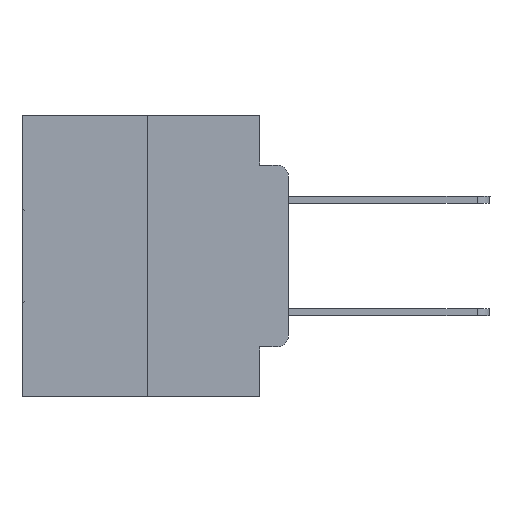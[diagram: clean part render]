
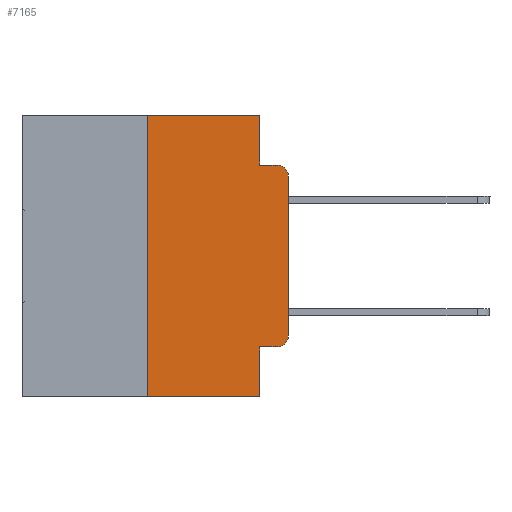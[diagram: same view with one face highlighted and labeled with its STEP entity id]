
A CAD part, left-side view. The second image highlights one B-rep face of the part: STEP entity #7165.
In plain terms, the highlighted planar face has unit normal (-1, 0, 0).
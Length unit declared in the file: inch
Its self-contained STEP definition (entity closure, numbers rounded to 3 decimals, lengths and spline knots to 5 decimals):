
#627 = CARTESIAN_POINT ( 'NONE',  ( 0., 0.25, 0. ) ) ;
#850 = DIRECTION ( 'NONE',  ( 0., 0., -1. ) ) ;
#1163 = LINE ( 'NONE', #29042, #15254 ) ;
#1243 = CARTESIAN_POINT ( 'NONE',  ( 0., 0., 0. ) ) ;
#1425 = DIRECTION ( 'NONE',  ( 1., 0., 0. ) ) ;
#1754 = VERTEX_POINT ( 'NONE', #24150 ) ;
#1997 = ORIENTED_EDGE ( 'NONE', *, *, #19515, .F. ) ;
#2080 = DIRECTION ( 'NONE',  ( 0., 0., 1. ) ) ;
#2230 = VERTEX_POINT ( 'NONE', #25196 ) ;
#2338 = ORIENTED_EDGE ( 'NONE', *, *, #7699, .T. ) ;
#2476 = LINE ( 'NONE', #18735, #23061 ) ;
#3043 = VERTEX_POINT ( 'NONE', #29175 ) ;
#3356 = VERTEX_POINT ( 'NONE', #10495 ) ;
#3398 = VECTOR ( 'NONE', #15623, 39.37008 ) ;
#3564 = LINE ( 'NONE', #5246, #29023 ) ;
#3790 = FACE_OUTER_BOUND ( 'NONE', #11510, .T. ) ;
#3826 = PLANE ( 'NONE',  #17827 ) ;
#3875 = EDGE_CURVE ( 'NONE', #5034, #3043, #18360, .T. ) ;
#4251 = VECTOR ( 'NONE', #21074, 39.37008 ) ;
#4512 = DIRECTION ( 'NONE',  ( 0., 0., -1. ) ) ;
#4772 = VECTOR ( 'NONE', #4512, 39.37008 ) ;
#4819 = CARTESIAN_POINT ( 'NONE',  ( 0., 0.25, 0. ) ) ;
#5034 = VERTEX_POINT ( 'NONE', #29821 ) ;
#5246 = CARTESIAN_POINT ( 'NONE',  ( 0., 0.051, -0.4115 ) ) ;
#5855 = ORIENTED_EDGE ( 'NONE', *, *, #11277, .T. ) ;
#6002 = CARTESIAN_POINT ( 'NONE',  ( 0., 0.473, -0.5 ) ) ;
#6087 = ORIENTED_EDGE ( 'NONE', *, *, #17859, .T. ) ;
#6363 = DIRECTION ( 'NONE',  ( 0., -1., 0. ) ) ;
#7165 = ADVANCED_FACE ( 'NONE', ( #3790 ), #3826, .F. ) ;
#7699 = EDGE_CURVE ( 'NONE', #14902, #1754, #9706, .T. ) ;
#8562 = CARTESIAN_POINT ( 'NONE',  ( 0., 0.051, -0.0885 ) ) ;
#8677 = CARTESIAN_POINT ( 'NONE',  ( 0., 0.051, -0.0885 ) ) ;
#8917 = CARTESIAN_POINT ( 'NONE',  ( 0., 0.473, 0. ) ) ;
#9706 = LINE ( 'NONE', #6002, #28449 ) ;
#10223 = CARTESIAN_POINT ( 'NONE',  ( 0., 0.051, -0.4115 ) ) ;
#10495 = CARTESIAN_POINT ( 'NONE',  ( 0., 0.02, -0.4115 ) ) ;
#11277 = EDGE_CURVE ( 'NONE', #3356, #5034, #25965, .T. ) ;
#11510 = EDGE_LOOP ( 'NONE', ( #21213, #19625, #21829, #30779, #28754, #30303, #2338, #1997, #6087, #5855 ) ) ;
#11858 = CARTESIAN_POINT ( 'NONE',  ( 0., 0.02, -0.1085 ) ) ;
#11973 = DIRECTION ( 'NONE',  ( 0., 0., -1. ) ) ;
#14324 = DIRECTION ( 'NONE',  ( 0., 0., -1. ) ) ;
#14902 = VERTEX_POINT ( 'NONE', #22316 ) ;
#15242 = EDGE_CURVE ( 'NONE', #29424, #2230, #2476, .T. ) ;
#15254 = VECTOR ( 'NONE', #11973, 39.37008 ) ;
#15623 = DIRECTION ( 'NONE',  ( 0., 0., 1. ) ) ;
#15851 = DIRECTION ( 'NONE',  ( -1., 0., 0. ) ) ;
#16694 = LINE ( 'NONE', #627, #3398 ) ;
#17188 = VERTEX_POINT ( 'NONE', #19169 ) ;
#17827 = AXIS2_PLACEMENT_3D ( 'NONE', #8917, #1425, #18847 ) ;
#17859 = EDGE_CURVE ( 'NONE', #21528, #3356, #3564, .T. ) ;
#18360 = LINE ( 'NONE', #1243, #31265 ) ;
#18735 = CARTESIAN_POINT ( 'NONE',  ( 0., 0.473, 0. ) ) ;
#18847 = DIRECTION ( 'NONE',  ( 0., 0., -1. ) ) ;
#19169 = CARTESIAN_POINT ( 'NONE',  ( 0., 0.02, -0.0885 ) ) ;
#19515 = EDGE_CURVE ( 'NONE', #21528, #1754, #1163, .T. ) ;
#19625 = ORIENTED_EDGE ( 'NONE', *, *, #29279, .T. ) ;
#20859 = DIRECTION ( 'NONE',  ( 0., -1., 0. ) ) ;
#21074 = DIRECTION ( 'NONE',  ( 0., -1., 0. ) ) ;
#21153 = EDGE_CURVE ( 'NONE', #14902, #29424, #16694, .T. ) ;
#21213 = ORIENTED_EDGE ( 'NONE', *, *, #3875, .T. ) ;
#21283 = VERTEX_POINT ( 'NONE', #8562 ) ;
#21528 = VERTEX_POINT ( 'NONE', #10223 ) ;
#21829 = ORIENTED_EDGE ( 'NONE', *, *, #27643, .F. ) ;
#21850 = CARTESIAN_POINT ( 'NONE',  ( 0., 0.051, 0. ) ) ;
#22316 = CARTESIAN_POINT ( 'NONE',  ( 0., 0.25, -0.5 ) ) ;
#22593 = DIRECTION ( 'NONE',  ( 0., -1., 0. ) ) ;
#23061 = VECTOR ( 'NONE', #6363, 39.37008 ) ;
#23289 = LINE ( 'NONE', #8677, #4251 ) ;
#24150 = CARTESIAN_POINT ( 'NONE',  ( 0., 0.051, -0.5 ) ) ;
#25196 = CARTESIAN_POINT ( 'NONE',  ( 0., 0.051, 0. ) ) ;
#25965 = CIRCLE ( 'NONE', #31102, 0.02 ) ;
#26047 = EDGE_CURVE ( 'NONE', #2230, #21283, #30893, .T. ) ;
#26588 = CIRCLE ( 'NONE', #26664, 0.02 ) ;
#26664 = AXIS2_PLACEMENT_3D ( 'NONE', #11858, #28934, #14324 ) ;
#27643 = EDGE_CURVE ( 'NONE', #21283, #17188, #23289, .T. ) ;
#28449 = VECTOR ( 'NONE', #20859, 39.37008 ) ;
#28754 = ORIENTED_EDGE ( 'NONE', *, *, #15242, .F. ) ;
#28934 = DIRECTION ( 'NONE',  ( -1., 0., 0. ) ) ;
#29023 = VECTOR ( 'NONE', #22593, 39.37008 ) ;
#29042 = CARTESIAN_POINT ( 'NONE',  ( 0., 0.051, 0. ) ) ;
#29175 = CARTESIAN_POINT ( 'NONE',  ( 0., 0., -0.1085 ) ) ;
#29279 = EDGE_CURVE ( 'NONE', #3043, #17188, #26588, .T. ) ;
#29424 = VERTEX_POINT ( 'NONE', #4819 ) ;
#29821 = CARTESIAN_POINT ( 'NONE',  ( 0., 0., -0.3915 ) ) ;
#30303 = ORIENTED_EDGE ( 'NONE', *, *, #21153, .F. ) ;
#30374 = CARTESIAN_POINT ( 'NONE',  ( 0., 0.02, -0.3915 ) ) ;
#30779 = ORIENTED_EDGE ( 'NONE', *, *, #26047, .F. ) ;
#30893 = LINE ( 'NONE', #21850, #4772 ) ;
#31102 = AXIS2_PLACEMENT_3D ( 'NONE', #30374, #15851, #850 ) ;
#31265 = VECTOR ( 'NONE', #2080, 39.37008 ) ;
